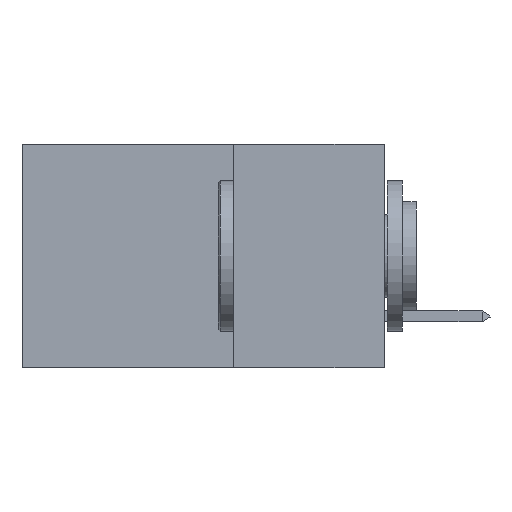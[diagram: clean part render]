
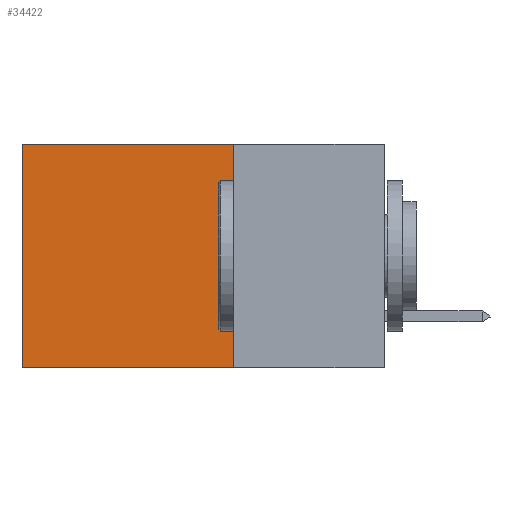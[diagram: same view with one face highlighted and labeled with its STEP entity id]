
A CAD part, left-side view. The second image highlights one B-rep face of the part: STEP entity #34422.
In plain terms, the highlighted planar face has unit normal (-1, 0, 0).
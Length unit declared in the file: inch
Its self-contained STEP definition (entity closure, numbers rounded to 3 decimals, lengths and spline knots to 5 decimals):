
#311 = FACE_OUTER_BOUND ( 'NONE', #25103, .T. ) ;
#1549 = CARTESIAN_POINT ( 'NONE',  ( 0.2875, 0.6, 0. ) ) ;
#4517 = VECTOR ( 'NONE', #10288, 39.37008 ) ;
#6079 = PLANE ( 'NONE',  #7548 ) ;
#7318 = CARTESIAN_POINT ( 'NONE',  ( 0.2875, 0.25, 0. ) ) ;
#7450 = DIRECTION ( 'NONE',  ( 0., 0., -1. ) ) ;
#7548 = AXIS2_PLACEMENT_3D ( 'NONE', #24892, #25023, #10064 ) ;
#10064 = DIRECTION ( 'NONE',  ( 0., 0., -1. ) ) ;
#10288 = DIRECTION ( 'NONE',  ( 0., 0., -1. ) ) ;
#11432 = EDGE_CURVE ( 'NONE', #29369, #39903, #13898, .T. ) ;
#12364 = CARTESIAN_POINT ( 'NONE',  ( 0.2875, 0.25, 0. ) ) ;
#12825 = CARTESIAN_POINT ( 'NONE',  ( 0.2875, 0.25, -0.37 ) ) ;
#12932 = EDGE_CURVE ( 'NONE', #29369, #32103, #27512, .T. ) ;
#13898 = LINE ( 'NONE', #7318, #40300 ) ;
#16325 = CARTESIAN_POINT ( 'NONE',  ( 0.2875, 0.25, -0.37 ) ) ;
#16518 = CARTESIAN_POINT ( 'NONE',  ( 0.2875, 0.6, 0. ) ) ;
#18580 = CARTESIAN_POINT ( 'NONE',  ( 0.2875, 0.25, 0. ) ) ;
#18727 = LINE ( 'NONE', #16518, #4517 ) ;
#21275 = VECTOR ( 'NONE', #28875, 39.37008 ) ;
#22189 = ORIENTED_EDGE ( 'NONE', *, *, #23976, .T. ) ;
#23976 = EDGE_CURVE ( 'NONE', #32103, #24152, #18727, .T. ) ;
#24152 = VERTEX_POINT ( 'NONE', #26499 ) ;
#24892 = CARTESIAN_POINT ( 'NONE',  ( 0.2875, 0.25, 0. ) ) ;
#25023 = DIRECTION ( 'NONE',  ( 1., 0., 0. ) ) ;
#25103 = EDGE_LOOP ( 'NONE', ( #22189, #30939, #39661, #35094 ) ) ;
#26499 = CARTESIAN_POINT ( 'NONE',  ( 0.2875, 0.6, -0.37 ) ) ;
#27111 = LINE ( 'NONE', #16325, #21275 ) ;
#27512 = LINE ( 'NONE', #12364, #37253 ) ;
#28875 = DIRECTION ( 'NONE',  ( 0., 1., 0. ) ) ;
#29369 = VERTEX_POINT ( 'NONE', #18580 ) ;
#30738 = EDGE_CURVE ( 'NONE', #39903, #24152, #27111, .T. ) ;
#30939 = ORIENTED_EDGE ( 'NONE', *, *, #30738, .F. ) ;
#32103 = VERTEX_POINT ( 'NONE', #1549 ) ;
#34422 = ADVANCED_FACE ( 'NONE', ( #311 ), #6079, .F. ) ;
#35094 = ORIENTED_EDGE ( 'NONE', *, *, #12932, .T. ) ;
#37078 = DIRECTION ( 'NONE',  ( 0., 1., 0. ) ) ;
#37253 = VECTOR ( 'NONE', #37078, 39.37008 ) ;
#39661 = ORIENTED_EDGE ( 'NONE', *, *, #11432, .F. ) ;
#39903 = VERTEX_POINT ( 'NONE', #12825 ) ;
#40300 = VECTOR ( 'NONE', #7450, 39.37008 ) ;
